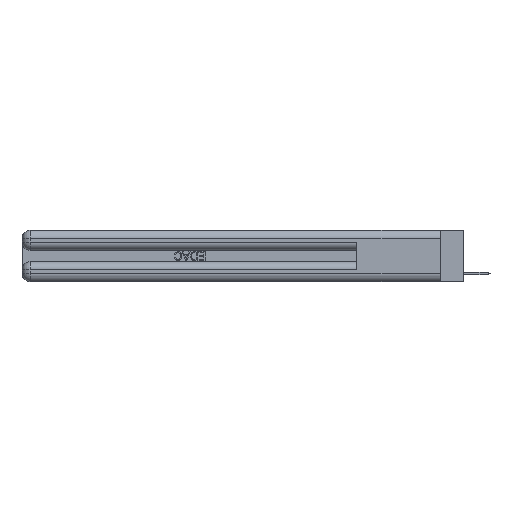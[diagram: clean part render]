
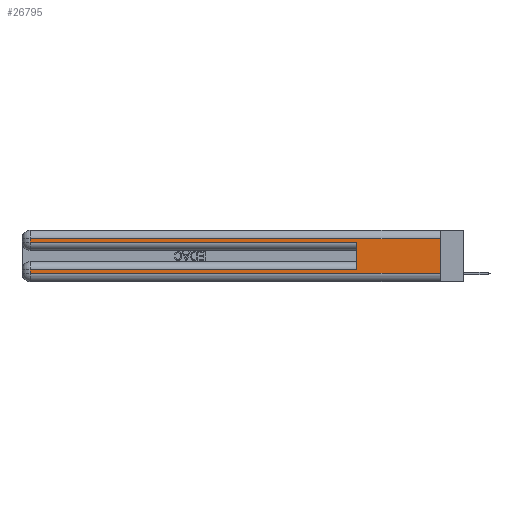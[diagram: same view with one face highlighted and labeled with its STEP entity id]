
A CAD part, left-side view. The second image highlights one B-rep face of the part: STEP entity #26795.
In plain terms, the highlighted planar face has unit normal (-1, 0, 0).
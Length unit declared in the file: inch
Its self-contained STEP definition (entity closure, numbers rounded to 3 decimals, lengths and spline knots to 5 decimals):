
#427 = DIRECTION ( 'NONE',  ( 0., 0., -1. ) ) ;
#583 = DIRECTION ( 'NONE',  ( 0., 0., -1. ) ) ;
#1361 = ORIENTED_EDGE ( 'NONE', *, *, #7283, .T. ) ;
#1365 = VERTEX_POINT ( 'NONE', #16310 ) ;
#1582 = VECTOR ( 'NONE', #21185, 39.37008 ) ;
#1939 = VERTEX_POINT ( 'NONE', #9477 ) ;
#2031 = EDGE_CURVE ( 'NONE', #20126, #3179, #10440, .T. ) ;
#3179 = VERTEX_POINT ( 'NONE', #15418 ) ;
#5505 = VECTOR ( 'NONE', #19801, 39.37008 ) ;
#6819 = CARTESIAN_POINT ( 'NONE',  ( 0., 0., 0.085 ) ) ;
#7283 = EDGE_CURVE ( 'NONE', #3179, #1939, #18274, .T. ) ;
#7832 = VERTEX_POINT ( 'NONE', #16459 ) ;
#7937 = CARTESIAN_POINT ( 'NONE',  ( 0., 2.94, 0.31 ) ) ;
#8460 = VECTOR ( 'NONE', #29103, 39.37008 ) ;
#8700 = PLANE ( 'NONE',  #15374 ) ;
#9477 = CARTESIAN_POINT ( 'NONE',  ( 0., 0.6, 0.285 ) ) ;
#9541 = VECTOR ( 'NONE', #19350, 39.37008 ) ;
#10440 = LINE ( 'NONE', #12853, #30412 ) ;
#10630 = ORIENTED_EDGE ( 'NONE', *, *, #22219, .F. ) ;
#10812 = VECTOR ( 'NONE', #31943, 39.37008 ) ;
#11393 = ORIENTED_EDGE ( 'NONE', *, *, #25164, .T. ) ;
#12853 = CARTESIAN_POINT ( 'NONE',  ( 0., 2.94, 0.37 ) ) ;
#13008 = ORIENTED_EDGE ( 'NONE', *, *, #22101, .F. ) ;
#13561 = CARTESIAN_POINT ( 'NONE',  ( 0., 0., 0.37 ) ) ;
#15374 = AXIS2_PLACEMENT_3D ( 'NONE', #13561, #21294, #16157 ) ;
#15418 = CARTESIAN_POINT ( 'NONE',  ( 0., 2.94, 0.285 ) ) ;
#16157 = DIRECTION ( 'NONE',  ( 0., 0., -1. ) ) ;
#16173 = VERTEX_POINT ( 'NONE', #23155 ) ;
#16308 = FACE_OUTER_BOUND ( 'NONE', #16672, .T. ) ;
#16310 = CARTESIAN_POINT ( 'NONE',  ( 0., 0., 0.31 ) ) ;
#16459 = CARTESIAN_POINT ( 'NONE',  ( 0., 2.94, 0.085 ) ) ;
#16521 = CARTESIAN_POINT ( 'NONE',  ( 0., 2.94, 0.37 ) ) ;
#16672 = EDGE_LOOP ( 'NONE', ( #10630, #23159, #31779, #1361, #13008, #31082, #11393, #26913 ) ) ;
#17874 = VECTOR ( 'NONE', #583, 39.37008 ) ;
#17882 = EDGE_CURVE ( 'NONE', #16173, #7832, #19236, .T. ) ;
#17963 = CARTESIAN_POINT ( 'NONE',  ( 0., 0., 0.285 ) ) ;
#18274 = LINE ( 'NONE', #17963, #30428 ) ;
#18504 = VERTEX_POINT ( 'NONE', #25332 ) ;
#19236 = LINE ( 'NONE', #6819, #8460 ) ;
#19350 = DIRECTION ( 'NONE',  ( 0., -1., 0. ) ) ;
#19801 = DIRECTION ( 'NONE',  ( 0., 0., 1. ) ) ;
#20126 = VERTEX_POINT ( 'NONE', #7937 ) ;
#20366 = EDGE_CURVE ( 'NONE', #23129, #18504, #22254, .T. ) ;
#21185 = DIRECTION ( 'NONE',  ( 0., 0., -1. ) ) ;
#21294 = DIRECTION ( 'NONE',  ( 1., 0., 0. ) ) ;
#21672 = LINE ( 'NONE', #16521, #1582 ) ;
#21798 = LINE ( 'NONE', #24718, #10812 ) ;
#22049 = LINE ( 'NONE', #24008, #5505 ) ;
#22101 = EDGE_CURVE ( 'NONE', #16173, #1939, #22049, .T. ) ;
#22219 = EDGE_CURVE ( 'NONE', #1365, #18504, #27713, .T. ) ;
#22254 = LINE ( 'NONE', #29380, #9541 ) ;
#22865 = CARTESIAN_POINT ( 'NONE',  ( 0., 0., 0.37 ) ) ;
#23129 = VERTEX_POINT ( 'NONE', #29527 ) ;
#23155 = CARTESIAN_POINT ( 'NONE',  ( 0., 0.6, 0.085 ) ) ;
#23159 = ORIENTED_EDGE ( 'NONE', *, *, #30678, .T. ) ;
#23442 = DIRECTION ( 'NONE',  ( 0., -1., 0. ) ) ;
#24008 = CARTESIAN_POINT ( 'NONE',  ( 0., 0.6, 0.145 ) ) ;
#24718 = CARTESIAN_POINT ( 'NONE',  ( 0., 0., 0.31 ) ) ;
#25164 = EDGE_CURVE ( 'NONE', #7832, #23129, #21672, .T. ) ;
#25332 = CARTESIAN_POINT ( 'NONE',  ( 0., 0., 0.06 ) ) ;
#26795 = ADVANCED_FACE ( 'NONE', ( #16308 ), #8700, .F. ) ;
#26913 = ORIENTED_EDGE ( 'NONE', *, *, #20366, .T. ) ;
#27713 = LINE ( 'NONE', #22865, #17874 ) ;
#29103 = DIRECTION ( 'NONE',  ( 0., 1., 0. ) ) ;
#29380 = CARTESIAN_POINT ( 'NONE',  ( 0., 0., 0.06 ) ) ;
#29527 = CARTESIAN_POINT ( 'NONE',  ( 0., 2.94, 0.06 ) ) ;
#30412 = VECTOR ( 'NONE', #427, 39.37008 ) ;
#30428 = VECTOR ( 'NONE', #23442, 39.37008 ) ;
#30678 = EDGE_CURVE ( 'NONE', #1365, #20126, #21798, .T. ) ;
#31082 = ORIENTED_EDGE ( 'NONE', *, *, #17882, .T. ) ;
#31779 = ORIENTED_EDGE ( 'NONE', *, *, #2031, .T. ) ;
#31943 = DIRECTION ( 'NONE',  ( 0., 1., 0. ) ) ;
